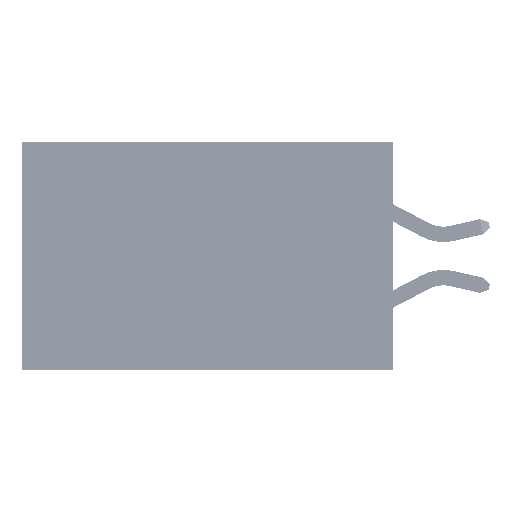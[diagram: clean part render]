
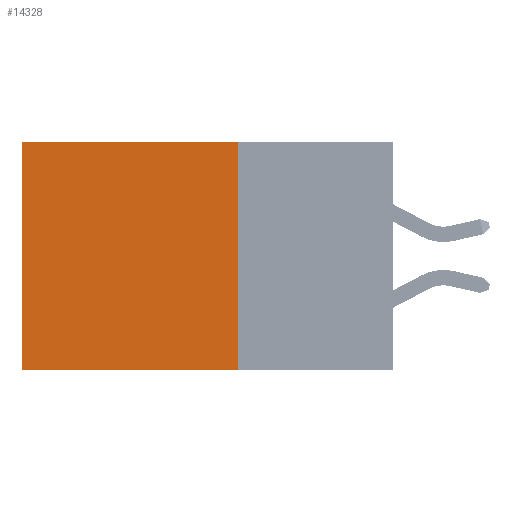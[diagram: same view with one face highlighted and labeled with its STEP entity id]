
A CAD part, left-side view. The second image highlights one B-rep face of the part: STEP entity #14328.
In plain terms, the highlighted planar face has unit normal (-1, 0, 0).
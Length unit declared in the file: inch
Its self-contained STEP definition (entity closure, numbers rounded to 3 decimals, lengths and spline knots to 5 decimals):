
#2289 = DIRECTION ( 'NONE',  ( 0., 0., -1. ) ) ;
#3849 = CARTESIAN_POINT ( 'NONE',  ( 0.2875, 0.6, -0.37 ) ) ;
#6066 = EDGE_LOOP ( 'NONE', ( #28990, #20143, #31298, #33328 ) ) ;
#8728 = VECTOR ( 'NONE', #39875, 39.37008 ) ;
#9134 = LINE ( 'NONE', #40644, #22228 ) ;
#9513 = FACE_OUTER_BOUND ( 'NONE', #6066, .T. ) ;
#9742 = VERTEX_POINT ( 'NONE', #41691 ) ;
#11377 = CARTESIAN_POINT ( 'NONE',  ( 0.2875, 0.25, -0.37 ) ) ;
#13709 = DIRECTION ( 'NONE',  ( 0., 0., -1. ) ) ;
#14328 = ADVANCED_FACE ( 'NONE', ( #9513 ), #46984, .F. ) ;
#15978 = EDGE_CURVE ( 'NONE', #29751, #9742, #33190, .T. ) ;
#16764 = CARTESIAN_POINT ( 'NONE',  ( 0.2875, 0.25, 0. ) ) ;
#17969 = EDGE_CURVE ( 'NONE', #9742, #30863, #9134, .T. ) ;
#20143 = ORIENTED_EDGE ( 'NONE', *, *, #38571, .F. ) ;
#20598 = DIRECTION ( 'NONE',  ( 1., 0., 0. ) ) ;
#20719 = CARTESIAN_POINT ( 'NONE',  ( 0.2875, 0.25, 0. ) ) ;
#20995 = CARTESIAN_POINT ( 'NONE',  ( 0.2875, 0.25, -0.37 ) ) ;
#22105 = VECTOR ( 'NONE', #13709, 39.37008 ) ;
#22228 = VECTOR ( 'NONE', #2289, 39.37008 ) ;
#24438 = DIRECTION ( 'NONE',  ( 0., 0., -1. ) ) ;
#28530 = VERTEX_POINT ( 'NONE', #11377 ) ;
#28990 = ORIENTED_EDGE ( 'NONE', *, *, #17969, .T. ) ;
#29390 = EDGE_CURVE ( 'NONE', #29751, #28530, #48386, .T. ) ;
#29600 = VECTOR ( 'NONE', #42421, 39.37008 ) ;
#29751 = VERTEX_POINT ( 'NONE', #42218 ) ;
#30863 = VERTEX_POINT ( 'NONE', #3849 ) ;
#31298 = ORIENTED_EDGE ( 'NONE', *, *, #29390, .F. ) ;
#33190 = LINE ( 'NONE', #38069, #29600 ) ;
#33328 = ORIENTED_EDGE ( 'NONE', *, *, #15978, .T. ) ;
#35871 = AXIS2_PLACEMENT_3D ( 'NONE', #16764, #20598, #24438 ) ;
#38069 = CARTESIAN_POINT ( 'NONE',  ( 0.2875, 0.25, 0. ) ) ;
#38571 = EDGE_CURVE ( 'NONE', #28530, #30863, #46376, .T. ) ;
#39875 = DIRECTION ( 'NONE',  ( 0., 1., 0. ) ) ;
#40644 = CARTESIAN_POINT ( 'NONE',  ( 0.2875, 0.6, 0. ) ) ;
#41691 = CARTESIAN_POINT ( 'NONE',  ( 0.2875, 0.6, 0. ) ) ;
#42218 = CARTESIAN_POINT ( 'NONE',  ( 0.2875, 0.25, 0. ) ) ;
#42421 = DIRECTION ( 'NONE',  ( 0., 1., 0. ) ) ;
#46376 = LINE ( 'NONE', #20995, #8728 ) ;
#46984 = PLANE ( 'NONE',  #35871 ) ;
#48386 = LINE ( 'NONE', #20719, #22105 ) ;
